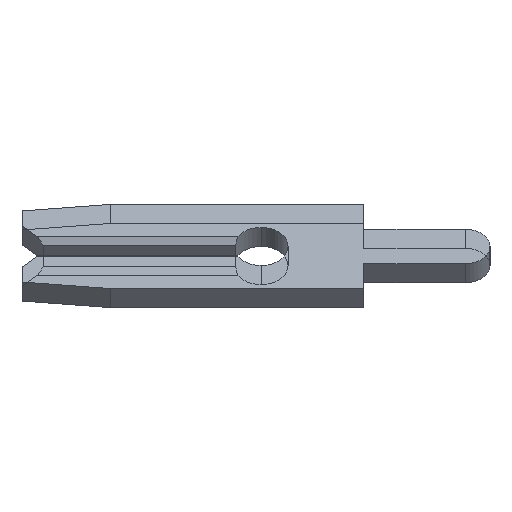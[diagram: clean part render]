
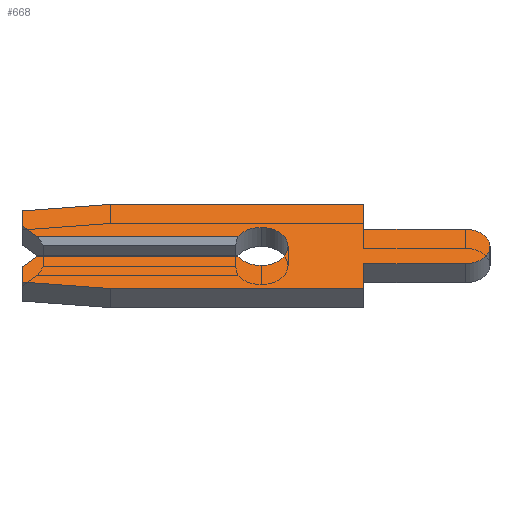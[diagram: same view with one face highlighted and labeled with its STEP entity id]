
A CAD part, left-side view. The second image highlights one B-rep face of the part: STEP entity #668.
In plain terms, the highlighted face is planar.
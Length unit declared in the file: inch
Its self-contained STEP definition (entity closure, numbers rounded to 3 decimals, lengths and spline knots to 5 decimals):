
#20 = LINE ( 'NONE', #1639, #2387 ) ;
#45 = CIRCLE ( 'NONE', #1954, 0.026 ) ;
#65 = CARTESIAN_POINT ( 'NONE',  ( -0.013, 0.146, -0.0575 ) ) ;
#108 = VECTOR ( 'NONE', #2429, 39.37008 ) ;
#116 = EDGE_CURVE ( 'NONE', #146, #755, #1477, .T. ) ;
#146 = VERTEX_POINT ( 'NONE', #2462 ) ;
#170 = PLANE ( 'NONE',  #631 ) ;
#183 = VERTEX_POINT ( 'NONE', #853 ) ;
#189 = EDGE_CURVE ( 'NONE', #816, #2495, #1927, .T. ) ;
#206 = ORIENTED_EDGE ( 'NONE', *, *, #2333, .F. ) ;
#218 = CARTESIAN_POINT ( 'NONE',  ( -0.013, 0.231, -0.028 ) ) ;
#226 = DIRECTION ( 'NONE',  ( 0., 0., 1. ) ) ;
#272 = EDGE_CURVE ( 'NONE', #880, #816, #360, .T. ) ;
#276 = DIRECTION ( 'NONE',  ( 0., 0.995, 0.105 ) ) ;
#297 = VERTEX_POINT ( 'NONE', #1087 ) ;
#319 = VECTOR ( 'NONE', #1472, 39.37008 ) ;
#334 = ORIENTED_EDGE ( 'NONE', *, *, #1916, .F. ) ;
#350 = VECTOR ( 'NONE', #457, 39.37008 ) ;
#360 = LINE ( 'NONE', #65, #319 ) ;
#366 = CARTESIAN_POINT ( 'NONE',  ( -0.013, 0., 0. ) ) ;
#395 = EDGE_LOOP ( 'NONE', ( #1859, #2277, #529, #554, #2243, #1866, #2339, #851, #2459, #206, #1636, #551, #1093, #2427, #1827, #334, #1696, #1792 ) ) ;
#398 = VERTEX_POINT ( 'NONE', #2307 ) ;
#399 = DIRECTION ( 'NONE',  ( 0., -0.995, 0.105 ) ) ;
#404 = DIRECTION ( 'NONE',  ( 0., 0., 1. ) ) ;
#414 = CARTESIAN_POINT ( 'NONE',  ( -0.013, -0.099, 0.0235 ) ) ;
#423 = DIRECTION ( 'NONE',  ( 0., 0., -1. ) ) ;
#429 = CARTESIAN_POINT ( 'NONE',  ( -0.013, -0.099, -0.0575 ) ) ;
#447 = LINE ( 'NONE', #945, #350 ) ;
#455 = CARTESIAN_POINT ( 'NONE',  ( -0.013, 0.231, -0.04857 ) ) ;
#457 = DIRECTION ( 'NONE',  ( 0., -1., 0. ) ) ;
#473 = DIRECTION ( 'NONE',  ( -1., 0., 0. ) ) ;
#477 = VECTOR ( 'NONE', #2414, 39.37008 ) ;
#484 = DIRECTION ( 'NONE',  ( 0., -1., 0. ) ) ;
#491 = VERTEX_POINT ( 'NONE', #1385 ) ;
#512 = LINE ( 'NONE', #2053, #477 ) ;
#529 = ORIENTED_EDGE ( 'NONE', *, *, #2469, .F. ) ;
#551 = ORIENTED_EDGE ( 'NONE', *, *, #2108, .F. ) ;
#554 = ORIENTED_EDGE ( 'NONE', *, *, #592, .F. ) ;
#556 = EDGE_CURVE ( 'NONE', #1193, #2159, #637, .T. ) ;
#562 = CARTESIAN_POINT ( 'NONE',  ( -0.013, 0.2105, 0.0075 ) ) ;
#565 = AXIS2_PLACEMENT_3D ( 'NONE', #2428, #1408, #404 ) ;
#592 = EDGE_CURVE ( 'NONE', #2096, #2083, #1808, .T. ) ;
#599 = DIRECTION ( 'NONE',  ( -1., 0., 0. ) ) ;
#614 = CARTESIAN_POINT ( 'NONE',  ( -0.013, -0.1975, 0.0235 ) ) ;
#623 = CARTESIAN_POINT ( 'NONE',  ( -0.013, -0.099, -0.0575 ) ) ;
#631 = AXIS2_PLACEMENT_3D ( 'NONE', #366, #2210, #986 ) ;
#633 = LINE ( 'NONE', #429, #2110 ) ;
#637 = LINE ( 'NONE', #1409, #108 ) ;
#668 = ADVANCED_FACE ( 'NONE', ( #1661 ), #170, .F. ) ;
#755 = VERTEX_POINT ( 'NONE', #614 ) ;
#770 = LINE ( 'NONE', #1017, #1841 ) ;
#810 = CARTESIAN_POINT ( 'NONE',  ( -0.013, 0., -0.026 ) ) ;
#816 = VERTEX_POINT ( 'NONE', #1831 ) ;
#851 = ORIENTED_EDGE ( 'NONE', *, *, #189, .F. ) ;
#853 = CARTESIAN_POINT ( 'NONE',  ( -0.013, -0.1975, -0.0235 ) ) ;
#880 = VERTEX_POINT ( 'NONE', #623 ) ;
#900 = VECTOR ( 'NONE', #2184, 39.37008 ) ;
#945 = CARTESIAN_POINT ( 'NONE',  ( -0.013, 0.146, 0.0575 ) ) ;
#964 = CARTESIAN_POINT ( 'NONE',  ( -0.013, 0.231, 0.04857 ) ) ;
#986 = DIRECTION ( 'NONE',  ( 0., 0., -1. ) ) ;
#1005 = DIRECTION ( 'NONE',  ( 0., 0., -1. ) ) ;
#1017 = CARTESIAN_POINT ( 'NONE',  ( -0.013, 0.231, 0.04857 ) ) ;
#1038 = DIRECTION ( 'NONE',  ( 0., -1., 0. ) ) ;
#1073 = CARTESIAN_POINT ( 'NONE',  ( -0.013, 0., 0.026 ) ) ;
#1076 = LINE ( 'NONE', #1384, #2014 ) ;
#1087 = CARTESIAN_POINT ( 'NONE',  ( -0.013, -0.099, -0.0235 ) ) ;
#1093 = ORIENTED_EDGE ( 'NONE', *, *, #116, .F. ) ;
#1138 = LINE ( 'NONE', #1698, #1653 ) ;
#1150 = VERTEX_POINT ( 'NONE', #2449 ) ;
#1171 = CIRCLE ( 'NONE', #565, 0.0235 ) ;
#1188 = CARTESIAN_POINT ( 'NONE',  ( -0.013, 0., 0. ) ) ;
#1193 = VERTEX_POINT ( 'NONE', #218 ) ;
#1213 = CARTESIAN_POINT ( 'NONE',  ( -0.013, 0., 0. ) ) ;
#1241 = EDGE_CURVE ( 'NONE', #2495, #1193, #1303, .T. ) ;
#1303 = LINE ( 'NONE', #2486, #1948 ) ;
#1312 = VERTEX_POINT ( 'NONE', #1073 ) ;
#1363 = VECTOR ( 'NONE', #226, 39.37008 ) ;
#1384 = CARTESIAN_POINT ( 'NONE',  ( -0.013, -0.099, -0.0235 ) ) ;
#1385 = CARTESIAN_POINT ( 'NONE',  ( -0.013, 0.231, 0.028 ) ) ;
#1395 = CARTESIAN_POINT ( 'NONE',  ( -0.013, 0.02252, -0.013 ) ) ;
#1408 = DIRECTION ( 'NONE',  ( 1., 0., 0. ) ) ;
#1409 = CARTESIAN_POINT ( 'NONE',  ( -0.013, 0.2105, -0.0075 ) ) ;
#1436 = EDGE_CURVE ( 'NONE', #1150, #1544, #447, .T. ) ;
#1464 = CARTESIAN_POINT ( 'NONE',  ( -0.013, 0.231, 0.028 ) ) ;
#1472 = DIRECTION ( 'NONE',  ( 0., 1., 0. ) ) ;
#1477 = LINE ( 'NONE', #414, #2299 ) ;
#1494 = DIRECTION ( 'NONE',  ( 0., 0., -1. ) ) ;
#1500 = CARTESIAN_POINT ( 'NONE',  ( -0.013, 0.231, -0.04857 ) ) ;
#1531 = VERTEX_POINT ( 'NONE', #1788 ) ;
#1544 = VERTEX_POINT ( 'NONE', #1765 ) ;
#1588 = DIRECTION ( 'NONE',  ( 0., 0., -1. ) ) ;
#1632 = VERTEX_POINT ( 'NONE', #964 ) ;
#1636 = ORIENTED_EDGE ( 'NONE', *, *, #1787, .F. ) ;
#1637 = AXIS2_PLACEMENT_3D ( 'NONE', #1188, #2425, #1588 ) ;
#1639 = CARTESIAN_POINT ( 'NONE',  ( -0.013, -0.099, 0.0575 ) ) ;
#1653 = VECTOR ( 'NONE', #484, 39.37008 ) ;
#1660 = EDGE_CURVE ( 'NONE', #398, #491, #2170, .T. ) ;
#1661 = FACE_OUTER_BOUND ( 'NONE', #395, .T. ) ;
#1696 = ORIENTED_EDGE ( 'NONE', *, *, #2136, .F. ) ;
#1698 = CARTESIAN_POINT ( 'NONE',  ( -0.013, 0.231, 0.013 ) ) ;
#1699 = EDGE_CURVE ( 'NONE', #2159, #2096, #512, .T. ) ;
#1719 = LINE ( 'NONE', #1464, #1363 ) ;
#1765 = CARTESIAN_POINT ( 'NONE',  ( -0.013, -0.099, 0.0575 ) ) ;
#1787 = EDGE_CURVE ( 'NONE', #183, #297, #1076, .T. ) ;
#1788 = CARTESIAN_POINT ( 'NONE',  ( -0.013, 0.02252, 0.013 ) ) ;
#1792 = ORIENTED_EDGE ( 'NONE', *, *, #1660, .F. ) ;
#1800 = DIRECTION ( 'NONE',  ( 0., 1., 0. ) ) ;
#1808 = CIRCLE ( 'NONE', #1637, 0.026 ) ;
#1827 = ORIENTED_EDGE ( 'NONE', *, *, #1436, .F. ) ;
#1831 = CARTESIAN_POINT ( 'NONE',  ( -0.013, 0.146, -0.0575 ) ) ;
#1841 = VECTOR ( 'NONE', #399, 39.37008 ) ;
#1855 = EDGE_CURVE ( 'NONE', #1312, #1531, #45, .T. ) ;
#1859 = ORIENTED_EDGE ( 'NONE', *, *, #2523, .T. ) ;
#1866 = ORIENTED_EDGE ( 'NONE', *, *, #556, .F. ) ;
#1894 = DIRECTION ( 'NONE',  ( 0., 0., 1. ) ) ;
#1916 = EDGE_CURVE ( 'NONE', #1632, #1150, #770, .T. ) ;
#1927 = LINE ( 'NONE', #455, #2032 ) ;
#1948 = VECTOR ( 'NONE', #1894, 39.37008 ) ;
#1954 = AXIS2_PLACEMENT_3D ( 'NONE', #1213, #599, #1005 ) ;
#1979 = CIRCLE ( 'NONE', #2087, 0.026 ) ;
#2014 = VECTOR ( 'NONE', #1800, 39.37008 ) ;
#2032 = VECTOR ( 'NONE', #276, 39.37008 ) ;
#2053 = CARTESIAN_POINT ( 'NONE',  ( -0.013, 0., -0.013 ) ) ;
#2059 = CARTESIAN_POINT ( 'NONE',  ( -0.013, 0.216, -0.013 ) ) ;
#2083 = VERTEX_POINT ( 'NONE', #810 ) ;
#2087 = AXIS2_PLACEMENT_3D ( 'NONE', #2301, #473, #1494 ) ;
#2096 = VERTEX_POINT ( 'NONE', #1395 ) ;
#2108 = EDGE_CURVE ( 'NONE', #755, #183, #1171, .T. ) ;
#2110 = VECTOR ( 'NONE', #2457, 39.37008 ) ;
#2136 = EDGE_CURVE ( 'NONE', #491, #1632, #1719, .T. ) ;
#2159 = VERTEX_POINT ( 'NONE', #2059 ) ;
#2170 = LINE ( 'NONE', #562, #900 ) ;
#2184 = DIRECTION ( 'NONE',  ( 0., 0.707, 0.707 ) ) ;
#2210 = DIRECTION ( 'NONE',  ( 1., 0., 0. ) ) ;
#2243 = ORIENTED_EDGE ( 'NONE', *, *, #1699, .F. ) ;
#2277 = ORIENTED_EDGE ( 'NONE', *, *, #1855, .F. ) ;
#2299 = VECTOR ( 'NONE', #1038, 39.37008 ) ;
#2301 = CARTESIAN_POINT ( 'NONE',  ( -0.013, 0., 0. ) ) ;
#2307 = CARTESIAN_POINT ( 'NONE',  ( -0.013, 0.216, 0.013 ) ) ;
#2316 = EDGE_CURVE ( 'NONE', #1544, #146, #20, .T. ) ;
#2333 = EDGE_CURVE ( 'NONE', #297, #880, #633, .T. ) ;
#2339 = ORIENTED_EDGE ( 'NONE', *, *, #1241, .F. ) ;
#2387 = VECTOR ( 'NONE', #423, 39.37008 ) ;
#2414 = DIRECTION ( 'NONE',  ( 0., -1., 0. ) ) ;
#2425 = DIRECTION ( 'NONE',  ( -1., 0., 0. ) ) ;
#2427 = ORIENTED_EDGE ( 'NONE', *, *, #2316, .F. ) ;
#2428 = CARTESIAN_POINT ( 'NONE',  ( -0.013, -0.1975, 0. ) ) ;
#2429 = DIRECTION ( 'NONE',  ( 0., -0.707, 0.707 ) ) ;
#2449 = CARTESIAN_POINT ( 'NONE',  ( -0.013, 0.146, 0.0575 ) ) ;
#2457 = DIRECTION ( 'NONE',  ( 0., 0., -1. ) ) ;
#2459 = ORIENTED_EDGE ( 'NONE', *, *, #272, .F. ) ;
#2462 = CARTESIAN_POINT ( 'NONE',  ( -0.013, -0.099, 0.0235 ) ) ;
#2469 = EDGE_CURVE ( 'NONE', #2083, #1312, #1979, .T. ) ;
#2486 = CARTESIAN_POINT ( 'NONE',  ( -0.013, 0.231, -0.028 ) ) ;
#2495 = VERTEX_POINT ( 'NONE', #1500 ) ;
#2523 = EDGE_CURVE ( 'NONE', #398, #1531, #1138, .T. ) ;
